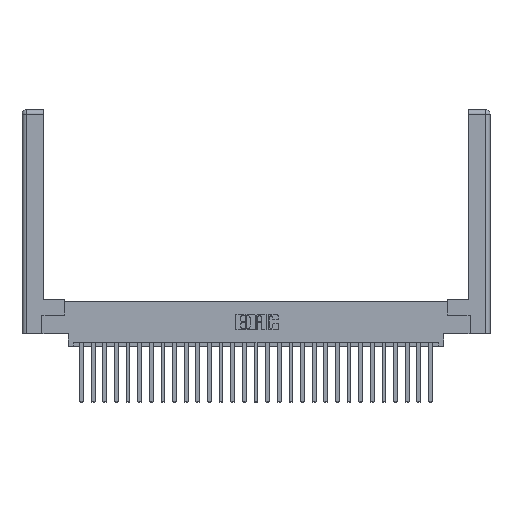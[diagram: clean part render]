
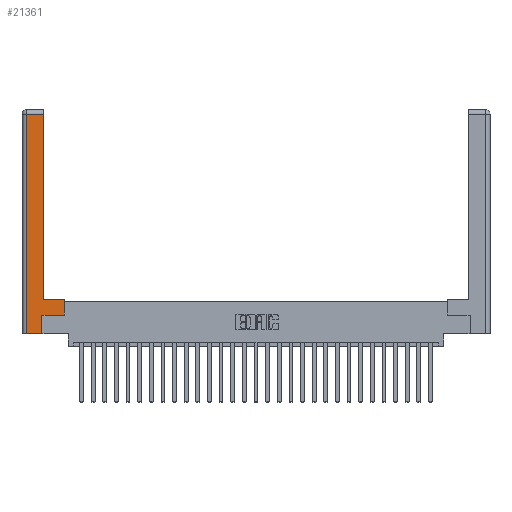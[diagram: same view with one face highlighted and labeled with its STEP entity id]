
A CAD part, top view. The second image highlights one B-rep face of the part: STEP entity #21361.
In plain terms, the highlighted planar face has unit normal (0, 0, 1).
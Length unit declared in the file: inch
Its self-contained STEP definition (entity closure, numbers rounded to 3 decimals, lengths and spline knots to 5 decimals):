
#259 = CARTESIAN_POINT ( 'NONE',  ( 0.265, 0.245, 0. ) ) ;
#823 = EDGE_CURVE ( 'NONE', #18947, #25586, #20110, .T. ) ;
#1222 = VERTEX_POINT ( 'NONE', #19961 ) ;
#2378 = LINE ( 'NONE', #10927, #15208 ) ;
#3513 = ORIENTED_EDGE ( 'NONE', *, *, #26130, .T. ) ;
#3543 = CARTESIAN_POINT ( 'NONE',  ( 0.295, 0.45, 0. ) ) ;
#3881 = EDGE_CURVE ( 'NONE', #1222, #11170, #23110, .T. ) ;
#4654 = CARTESIAN_POINT ( 'NONE',  ( 0.0615, 0., 0. ) ) ;
#5248 = DIRECTION ( 'NONE',  ( -1., 0., 0. ) ) ;
#5264 = CARTESIAN_POINT ( 'NONE',  ( 0.265, 0., 0. ) ) ;
#5895 = VECTOR ( 'NONE', #14737, 39.37008 ) ;
#5898 = EDGE_CURVE ( 'NONE', #15298, #18947, #2378, .T. ) ;
#6350 = EDGE_CURVE ( 'NONE', #15691, #1222, #8931, .T. ) ;
#6431 = ORIENTED_EDGE ( 'NONE', *, *, #12635, .T. ) ;
#6881 = VECTOR ( 'NONE', #23365, 39.37008 ) ;
#7370 = LINE ( 'NONE', #23624, #21207 ) ;
#8401 = EDGE_LOOP ( 'NONE', ( #13766, #3513, #12471, #13135, #22768, #9935, #12179, #6431 ) ) ;
#8931 = LINE ( 'NONE', #23730, #6881 ) ;
#9763 = VERTEX_POINT ( 'NONE', #24624 ) ;
#9935 = ORIENTED_EDGE ( 'NONE', *, *, #6350, .T. ) ;
#10058 = CARTESIAN_POINT ( 'NONE',  ( 0.295, 3., 0. ) ) ;
#10927 = CARTESIAN_POINT ( 'NONE',  ( 0.0615, 0., 0. ) ) ;
#10979 = EDGE_CURVE ( 'NONE', #9763, #27227, #22209, .T. ) ;
#11142 = FACE_OUTER_BOUND ( 'NONE', #8401, .T. ) ;
#11170 = VERTEX_POINT ( 'NONE', #24356 ) ;
#12179 = ORIENTED_EDGE ( 'NONE', *, *, #3881, .T. ) ;
#12471 = ORIENTED_EDGE ( 'NONE', *, *, #5898, .T. ) ;
#12635 = EDGE_CURVE ( 'NONE', #11170, #9763, #14176, .T. ) ;
#13135 = ORIENTED_EDGE ( 'NONE', *, *, #823, .T. ) ;
#13259 = DIRECTION ( 'NONE',  ( 0., 1., 0. ) ) ;
#13766 = ORIENTED_EDGE ( 'NONE', *, *, #10979, .T. ) ;
#13868 = CARTESIAN_POINT ( 'NONE',  ( 0.295, 2.94, 0. ) ) ;
#14176 = LINE ( 'NONE', #3543, #26791 ) ;
#14737 = DIRECTION ( 'NONE',  ( 1., 0., 0. ) ) ;
#15208 = VECTOR ( 'NONE', #15460, 39.37008 ) ;
#15298 = VERTEX_POINT ( 'NONE', #27212 ) ;
#15326 = CARTESIAN_POINT ( 'NONE',  ( 0.265, 0.245, 0. ) ) ;
#15361 = DIRECTION ( 'NONE',  ( 0., 1., 0. ) ) ;
#15460 = DIRECTION ( 'NONE',  ( 0., -1., 0. ) ) ;
#15691 = VERTEX_POINT ( 'NONE', #15326 ) ;
#16183 = DIRECTION ( 'NONE',  ( -1., 0., 0. ) ) ;
#16364 = VECTOR ( 'NONE', #13259, 39.37008 ) ;
#16461 = VECTOR ( 'NONE', #18557, 39.37008 ) ;
#17020 = DIRECTION ( 'NONE',  ( -1., 0., 0. ) ) ;
#17790 = DIRECTION ( 'NONE',  ( 0., 0., -1. ) ) ;
#18461 = VECTOR ( 'NONE', #15361, 39.37008 ) ;
#18557 = DIRECTION ( 'NONE',  ( 0., 1., 0. ) ) ;
#18947 = VERTEX_POINT ( 'NONE', #4654 ) ;
#19205 = LINE ( 'NONE', #259, #18461 ) ;
#19961 = CARTESIAN_POINT ( 'NONE',  ( 0.565, 0.245, 0. ) ) ;
#20110 = LINE ( 'NONE', #20986, #5895 ) ;
#20986 = CARTESIAN_POINT ( 'NONE',  ( 0.265, 0., 0. ) ) ;
#21207 = VECTOR ( 'NONE', #17020, 39.37008 ) ;
#21361 = ADVANCED_FACE ( 'NONE', ( #11142 ), #24561, .F. ) ;
#22209 = LINE ( 'NONE', #10058, #16461 ) ;
#22435 = CARTESIAN_POINT ( 'NONE',  ( 0., 0., 0. ) ) ;
#22660 = CARTESIAN_POINT ( 'NONE',  ( 0.565, 0.45, 0. ) ) ;
#22768 = ORIENTED_EDGE ( 'NONE', *, *, #25469, .T. ) ;
#23110 = LINE ( 'NONE', #22660, #16364 ) ;
#23365 = DIRECTION ( 'NONE',  ( 1., 0., 0. ) ) ;
#23624 = CARTESIAN_POINT ( 'NONE',  ( 0.0615, 2.94, 0. ) ) ;
#23730 = CARTESIAN_POINT ( 'NONE',  ( 0.565, 0.245, 0. ) ) ;
#24356 = CARTESIAN_POINT ( 'NONE',  ( 0.565, 0.45, 0. ) ) ;
#24561 = PLANE ( 'NONE',  #27475 ) ;
#24624 = CARTESIAN_POINT ( 'NONE',  ( 0.295, 0.45, 0. ) ) ;
#25469 = EDGE_CURVE ( 'NONE', #25586, #15691, #19205, .T. ) ;
#25586 = VERTEX_POINT ( 'NONE', #5264 ) ;
#26130 = EDGE_CURVE ( 'NONE', #27227, #15298, #7370, .T. ) ;
#26791 = VECTOR ( 'NONE', #16183, 39.37008 ) ;
#27212 = CARTESIAN_POINT ( 'NONE',  ( 0.0615, 2.94, 0. ) ) ;
#27227 = VERTEX_POINT ( 'NONE', #13868 ) ;
#27475 = AXIS2_PLACEMENT_3D ( 'NONE', #22435, #17790, #5248 ) ;
